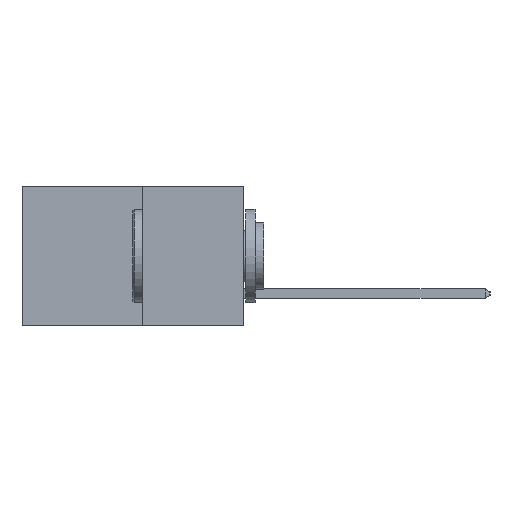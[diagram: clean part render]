
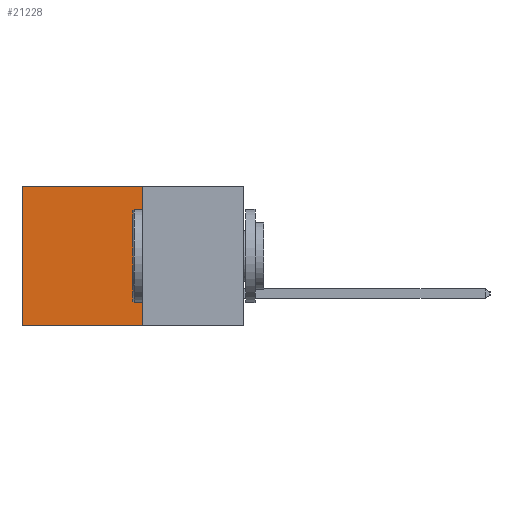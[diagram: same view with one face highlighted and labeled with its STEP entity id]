
A CAD part, left-side view. The second image highlights one B-rep face of the part: STEP entity #21228.
In plain terms, the highlighted planar face has unit normal (-1, 0, 0).
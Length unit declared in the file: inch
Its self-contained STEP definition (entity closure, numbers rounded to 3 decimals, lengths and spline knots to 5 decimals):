
#798 = VERTEX_POINT ( 'NONE', #2852 ) ;
#1354 = CARTESIAN_POINT ( 'NONE',  ( 0.277, 0.59, 0. ) ) ;
#2852 = CARTESIAN_POINT ( 'NONE',  ( 0.277, 0.27, -0.37 ) ) ;
#3983 = VECTOR ( 'NONE', #6557, 39.37008 ) ;
#4544 = CARTESIAN_POINT ( 'NONE',  ( 0.277, 0.59, -0.37 ) ) ;
#5952 = VERTEX_POINT ( 'NONE', #1354 ) ;
#6445 = VECTOR ( 'NONE', #25651, 39.37008 ) ;
#6528 = VECTOR ( 'NONE', #24714, 39.37008 ) ;
#6557 = DIRECTION ( 'NONE',  ( 0., 1., 0. ) ) ;
#8103 = VERTEX_POINT ( 'NONE', #12228 ) ;
#9516 = CARTESIAN_POINT ( 'NONE',  ( 0.277, 0.59, -0.37 ) ) ;
#9912 = ORIENTED_EDGE ( 'NONE', *, *, #24820, .F. ) ;
#9960 = CARTESIAN_POINT ( 'NONE',  ( 0.277, 0.27, 0. ) ) ;
#11940 = EDGE_CURVE ( 'NONE', #798, #15199, #15039, .T. ) ;
#12228 = CARTESIAN_POINT ( 'NONE',  ( 0.277, 0.27, 0. ) ) ;
#12383 = CARTESIAN_POINT ( 'NONE',  ( 0.277, 0.27, -0.37 ) ) ;
#13256 = LINE ( 'NONE', #4544, #6528 ) ;
#14335 = CARTESIAN_POINT ( 'NONE',  ( 0.277, 0.27, -0.37 ) ) ;
#14755 = DIRECTION ( 'NONE',  ( 0., 0., -1. ) ) ;
#15039 = LINE ( 'NONE', #15544, #3983 ) ;
#15199 = VERTEX_POINT ( 'NONE', #9516 ) ;
#15213 = FACE_OUTER_BOUND ( 'NONE', #19485, .T. ) ;
#15544 = CARTESIAN_POINT ( 'NONE',  ( 0.277, 0.27, -0.37 ) ) ;
#16740 = VECTOR ( 'NONE', #27702, 39.37008 ) ;
#18820 = ORIENTED_EDGE ( 'NONE', *, *, #11940, .F. ) ;
#19485 = EDGE_LOOP ( 'NONE', ( #23864, #18820, #9912, #22642 ) ) ;
#21228 = ADVANCED_FACE ( 'NONE', ( #15213 ), #25909, .F. ) ;
#22642 = ORIENTED_EDGE ( 'NONE', *, *, #25899, .T. ) ;
#22970 = LINE ( 'NONE', #9960, #6445 ) ;
#23864 = ORIENTED_EDGE ( 'NONE', *, *, #24572, .T. ) ;
#24572 = EDGE_CURVE ( 'NONE', #5952, #15199, #13256, .T. ) ;
#24714 = DIRECTION ( 'NONE',  ( 0., 0., -1. ) ) ;
#24820 = EDGE_CURVE ( 'NONE', #8103, #798, #28559, .T. ) ;
#25651 = DIRECTION ( 'NONE',  ( 0., 1., 0. ) ) ;
#25899 = EDGE_CURVE ( 'NONE', #8103, #5952, #22970, .T. ) ;
#25909 = PLANE ( 'NONE',  #26702 ) ;
#26702 = AXIS2_PLACEMENT_3D ( 'NONE', #12383, #28091, #14755 ) ;
#27702 = DIRECTION ( 'NONE',  ( 0., 0., -1. ) ) ;
#28091 = DIRECTION ( 'NONE',  ( 1., 0., 0. ) ) ;
#28559 = LINE ( 'NONE', #14335, #16740 ) ;
